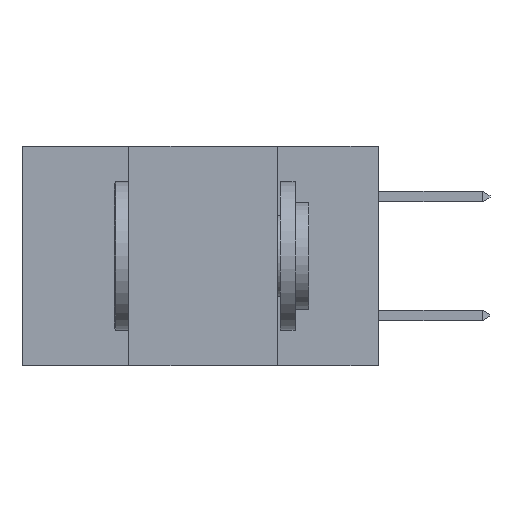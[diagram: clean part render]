
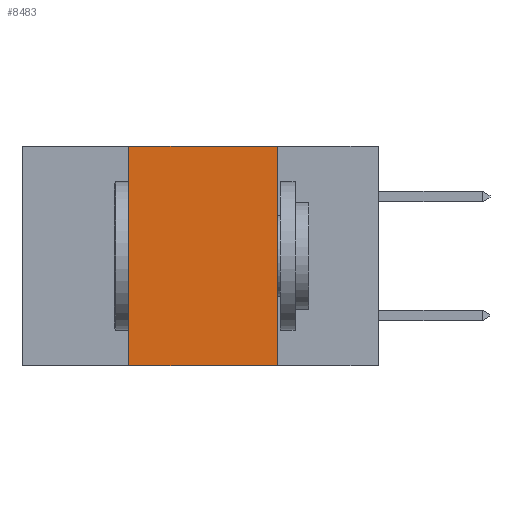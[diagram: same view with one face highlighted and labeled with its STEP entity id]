
A CAD part, left-side view. The second image highlights one B-rep face of the part: STEP entity #8483.
In plain terms, the highlighted planar face has unit normal (-1, 0, 0).
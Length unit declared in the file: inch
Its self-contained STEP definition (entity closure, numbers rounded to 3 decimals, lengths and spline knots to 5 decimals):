
#453 = CARTESIAN_POINT ( 'NONE',  ( 0., 0.42, 0. ) ) ;
#1320 = CARTESIAN_POINT ( 'NONE',  ( 0., 0.6, 0. ) ) ;
#1722 = EDGE_CURVE ( 'NONE', #5592, #23787, #10137, .T. ) ;
#1932 = EDGE_CURVE ( 'NONE', #25628, #5592, #10458, .T. ) ;
#2275 = CARTESIAN_POINT ( 'NONE',  ( 0., 0.17, 0. ) ) ;
#2366 = ORIENTED_EDGE ( 'NONE', *, *, #1932, .F. ) ;
#3051 = DIRECTION ( 'NONE',  ( 0., 0., 1. ) ) ;
#4743 = LINE ( 'NONE', #13171, #11012 ) ;
#4858 = VECTOR ( 'NONE', #18361, 39.37008 ) ;
#5592 = VERTEX_POINT ( 'NONE', #2275 ) ;
#6023 = PLANE ( 'NONE',  #17411 ) ;
#7743 = EDGE_CURVE ( 'NONE', #22990, #25628, #23618, .T. ) ;
#8124 = ORIENTED_EDGE ( 'NONE', *, *, #7743, .F. ) ;
#8483 = ADVANCED_FACE ( 'NONE', ( #26536 ), #6023, .F. ) ;
#10137 = LINE ( 'NONE', #16862, #26026 ) ;
#10271 = CARTESIAN_POINT ( 'NONE',  ( 0., 0.6, 0. ) ) ;
#10458 = LINE ( 'NONE', #1320, #4858 ) ;
#11012 = VECTOR ( 'NONE', #15234, 39.37008 ) ;
#12435 = DIRECTION ( 'NONE',  ( 0., 0., -1. ) ) ;
#13171 = CARTESIAN_POINT ( 'NONE',  ( 0., 0.6, -0.37 ) ) ;
#15234 = DIRECTION ( 'NONE',  ( 0., -1., 0. ) ) ;
#16048 = DIRECTION ( 'NONE',  ( 0., 0., -1. ) ) ;
#16862 = CARTESIAN_POINT ( 'NONE',  ( 0., 0.17, 0. ) ) ;
#17411 = AXIS2_PLACEMENT_3D ( 'NONE', #10271, #24766, #12435 ) ;
#18361 = DIRECTION ( 'NONE',  ( 0., -1., 0. ) ) ;
#18478 = ORIENTED_EDGE ( 'NONE', *, *, #19274, .T. ) ;
#19274 = EDGE_CURVE ( 'NONE', #22990, #23787, #4743, .T. ) ;
#19667 = CARTESIAN_POINT ( 'NONE',  ( 0., 0.42, -0.37 ) ) ;
#22977 = VECTOR ( 'NONE', #3051, 39.37008 ) ;
#22990 = VERTEX_POINT ( 'NONE', #19667 ) ;
#23618 = LINE ( 'NONE', #453, #22977 ) ;
#23787 = VERTEX_POINT ( 'NONE', #24908 ) ;
#24552 = CARTESIAN_POINT ( 'NONE',  ( 0., 0.42, 0. ) ) ;
#24766 = DIRECTION ( 'NONE',  ( 1., 0., 0. ) ) ;
#24908 = CARTESIAN_POINT ( 'NONE',  ( 0., 0.17, -0.37 ) ) ;
#25628 = VERTEX_POINT ( 'NONE', #24552 ) ;
#25907 = EDGE_LOOP ( 'NONE', ( #26778, #2366, #8124, #18478 ) ) ;
#26026 = VECTOR ( 'NONE', #16048, 39.37008 ) ;
#26536 = FACE_OUTER_BOUND ( 'NONE', #25907, .T. ) ;
#26778 = ORIENTED_EDGE ( 'NONE', *, *, #1722, .F. ) ;
